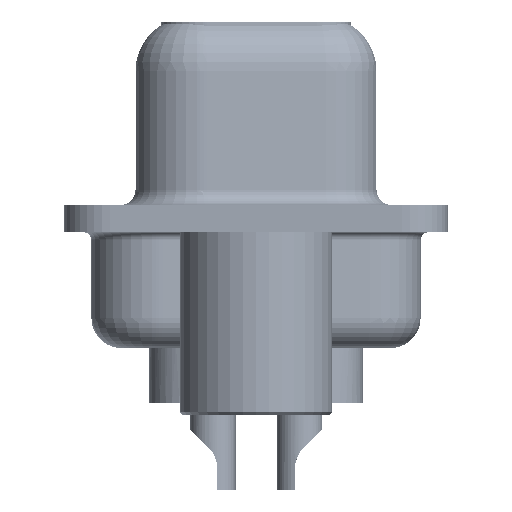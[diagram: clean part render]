
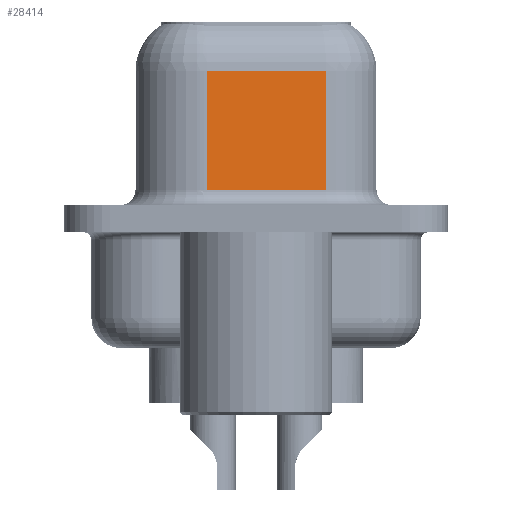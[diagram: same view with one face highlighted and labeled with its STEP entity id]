
A CAD part, left-side view. The second image highlights one B-rep face of the part: STEP entity #28414.
In plain terms, the highlighted planar face has unit normal (-0.985, -0.174, 0).
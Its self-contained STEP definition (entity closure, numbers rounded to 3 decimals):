
#93 = CARTESIAN_POINT ( 'NONE',  ( 5.068, -2.297, 4.85 ) ) ;
#1522 = FACE_OUTER_BOUND ( 'NONE', #22482, .T. ) ;
#1563 = CARTESIAN_POINT ( 'NONE',  ( 5.068, -2.297, 0.95 ) ) ;
#2537 = VECTOR ( 'NONE', #22606, 1000. ) ;
#4256 = EDGE_CURVE ( 'NONE', #19132, #9865, #14611, .T. ) ;
#5023 = CARTESIAN_POINT ( 'NONE',  ( 4.38, 1.603, 6.6 ) ) ;
#6509 = LINE ( 'NONE', #15868, #15990 ) ;
#8389 = PLANE ( 'NONE',  #13463 ) ;
#8701 = DIRECTION ( 'NONE',  ( 0., 0., -1. ) ) ;
#9865 = VERTEX_POINT ( 'NONE', #16088 ) ;
#10604 = VERTEX_POINT ( 'NONE', #19603 ) ;
#10669 = CARTESIAN_POINT ( 'NONE',  ( 5.068, -2.297, 4.85 ) ) ;
#11144 = ORIENTED_EDGE ( 'NONE', *, *, #4256, .T. ) ;
#11278 = VECTOR ( 'NONE', #29115, 1000. ) ;
#12156 = CARTESIAN_POINT ( 'NONE',  ( 4.38, 1.603, 0.95 ) ) ;
#12599 = ORIENTED_EDGE ( 'NONE', *, *, #15270, .T. ) ;
#13463 = AXIS2_PLACEMENT_3D ( 'NONE', #20546, #13689, #20844 ) ;
#13630 = EDGE_CURVE ( 'NONE', #19132, #10604, #6509, .T. ) ;
#13689 = DIRECTION ( 'NONE',  ( 0.985, 0.174, 0. ) ) ;
#14611 = LINE ( 'NONE', #93, #11278 ) ;
#15270 = EDGE_CURVE ( 'NONE', #18268, #10604, #25121, .T. ) ;
#15868 = CARTESIAN_POINT ( 'NONE',  ( 5.068, -2.297, 6.6 ) ) ;
#15990 = VECTOR ( 'NONE', #8701, 1000. ) ;
#16088 = CARTESIAN_POINT ( 'NONE',  ( 4.38, 1.603, 4.85 ) ) ;
#17030 = LINE ( 'NONE', #5023, #26684 ) ;
#18268 = VERTEX_POINT ( 'NONE', #12156 ) ;
#18562 = ORIENTED_EDGE ( 'NONE', *, *, #13630, .F. ) ;
#18882 = DIRECTION ( 'NONE',  ( 0., 0., -1. ) ) ;
#19132 = VERTEX_POINT ( 'NONE', #10669 ) ;
#19603 = CARTESIAN_POINT ( 'NONE',  ( 5.068, -2.297, 0.95 ) ) ;
#20546 = CARTESIAN_POINT ( 'NONE',  ( 5.068, -2.297, 6.6 ) ) ;
#20825 = EDGE_CURVE ( 'NONE', #9865, #18268, #17030, .T. ) ;
#20844 = DIRECTION ( 'NONE',  ( -0.174, 0.985, 0. ) ) ;
#22482 = EDGE_LOOP ( 'NONE', ( #18562, #11144, #23316, #12599 ) ) ;
#22606 = DIRECTION ( 'NONE',  ( 0.174, -0.985, 0. ) ) ;
#23316 = ORIENTED_EDGE ( 'NONE', *, *, #20825, .T. ) ;
#25121 = LINE ( 'NONE', #1563, #2537 ) ;
#26684 = VECTOR ( 'NONE', #18882, 1000. ) ;
#28414 = ADVANCED_FACE ( 'NONE', ( #1522 ), #8389, .F. ) ;
#29115 = DIRECTION ( 'NONE',  ( -0.174, 0.985, 0. ) ) ;
